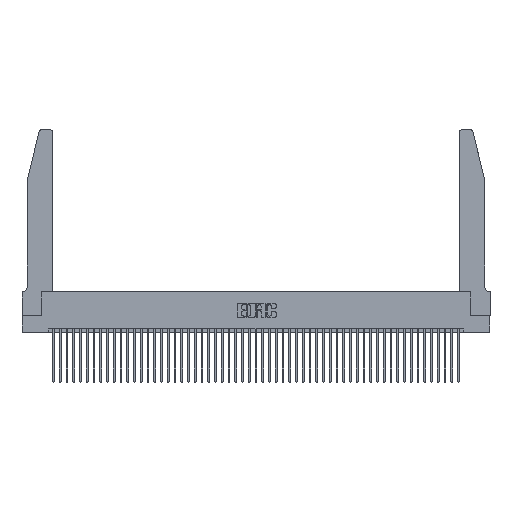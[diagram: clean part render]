
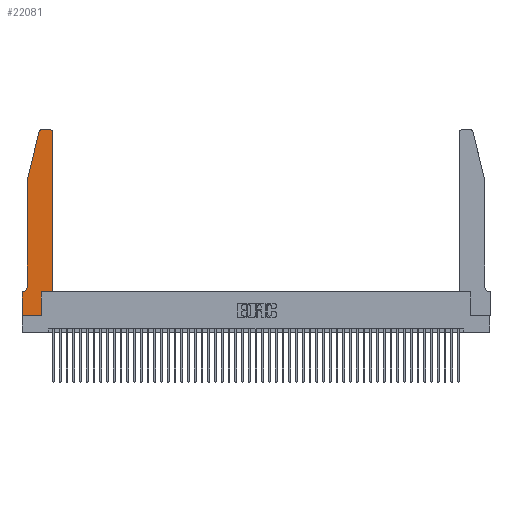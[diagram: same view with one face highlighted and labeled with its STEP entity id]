
A CAD part, top view. The second image highlights one B-rep face of the part: STEP entity #22081.
In plain terms, the highlighted planar face has unit normal (0, 0, 1).
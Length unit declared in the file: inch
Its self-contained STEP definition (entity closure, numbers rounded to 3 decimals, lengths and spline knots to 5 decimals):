
#239 = DIRECTION ( 'NONE',  ( -1., 0., 0. ) ) ;
#537 = CARTESIAN_POINT ( 'NONE',  ( 0.0755, 2., 0.37 ) ) ;
#683 = EDGE_CURVE ( 'NONE', #21842, #46293, #47460, .T. ) ;
#804 = AXIS2_PLACEMENT_3D ( 'NONE', #44240, #5636, #13588 ) ;
#1028 = VERTEX_POINT ( 'NONE', #24618 ) ;
#1749 = VECTOR ( 'NONE', #37568, 39.37008 ) ;
#1905 = EDGE_CURVE ( 'NONE', #1028, #19349, #47567, .T. ) ;
#2103 = ORIENTED_EDGE ( 'NONE', *, *, #21522, .T. ) ;
#2337 = DIRECTION ( 'NONE',  ( 0., 0., 1. ) ) ;
#2637 = CIRCLE ( 'NONE', #40238, 0.03 ) ;
#3831 = VERTEX_POINT ( 'NONE', #17701 ) ;
#4755 = LINE ( 'NONE', #44867, #1749 ) ;
#5112 = CIRCLE ( 'NONE', #804, 0.07 ) ;
#5511 = VECTOR ( 'NONE', #21574, 39.37008 ) ;
#5636 = DIRECTION ( 'NONE',  ( 0., 0., -1. ) ) ;
#5641 = LINE ( 'NONE', #6228, #22602 ) ;
#5674 = VECTOR ( 'NONE', #14822, 39.37008 ) ;
#5679 = CARTESIAN_POINT ( 'NONE',  ( 0.2865, 0.35, 0.37 ) ) ;
#6228 = CARTESIAN_POINT ( 'NONE',  ( 0.4505, 0.35, 0.37 ) ) ;
#7110 = ORIENTED_EDGE ( 'NONE', *, *, #42096, .T. ) ;
#7933 = VERTEX_POINT ( 'NONE', #45067 ) ;
#8116 = VERTEX_POINT ( 'NONE', #537 ) ;
#8693 = ORIENTED_EDGE ( 'NONE', *, *, #1905, .T. ) ;
#8841 = ORIENTED_EDGE ( 'NONE', *, *, #12500, .T. ) ;
#9583 = CARTESIAN_POINT ( 'NONE',  ( 0.4505, 0.35, 0.37 ) ) ;
#9733 = CARTESIAN_POINT ( 'NONE',  ( 0.2865, 0., 0.37 ) ) ;
#9980 = LINE ( 'NONE', #12055, #46241 ) ;
#10110 = VERTEX_POINT ( 'NONE', #5679 ) ;
#10448 = DIRECTION ( 'NONE',  ( 1., 0., 0. ) ) ;
#10725 = CARTESIAN_POINT ( 'NONE',  ( 0., 0.35, 0.37 ) ) ;
#11738 = VECTOR ( 'NONE', #10448, 39.37008 ) ;
#12055 = CARTESIAN_POINT ( 'NONE',  ( 0.0755, 0.35, 0.37 ) ) ;
#12152 = ORIENTED_EDGE ( 'NONE', *, *, #33700, .T. ) ;
#12319 = EDGE_CURVE ( 'NONE', #37560, #8116, #18363, .T. ) ;
#12500 = EDGE_CURVE ( 'NONE', #10110, #3831, #5641, .T. ) ;
#13588 = DIRECTION ( 'NONE',  ( -1., 0., 0. ) ) ;
#13755 = AXIS2_PLACEMENT_3D ( 'NONE', #10725, #14436, #45393 ) ;
#14143 = VECTOR ( 'NONE', #43147, 39.37008 ) ;
#14239 = ORIENTED_EDGE ( 'NONE', *, *, #46675, .T. ) ;
#14299 = LINE ( 'NONE', #9583, #16076 ) ;
#14436 = DIRECTION ( 'NONE',  ( 0., 0., 1. ) ) ;
#14731 = DIRECTION ( 'NONE',  ( 1., 0., 0. ) ) ;
#14822 = DIRECTION ( 'NONE',  ( 0., -1., 0. ) ) ;
#15952 = VERTEX_POINT ( 'NONE', #25430 ) ;
#16050 = CARTESIAN_POINT ( 'NONE',  ( 0.0755, 2., 0.37 ) ) ;
#16076 = VECTOR ( 'NONE', #17682, 39.37008 ) ;
#16560 = CARTESIAN_POINT ( 'NONE',  ( 0.2865, 0.35, 0.37 ) ) ;
#17682 = DIRECTION ( 'NONE',  ( 0., 1., 0. ) ) ;
#17701 = CARTESIAN_POINT ( 'NONE',  ( 0.4505, 0.35, 0.37 ) ) ;
#18363 = LINE ( 'NONE', #16050, #14143 ) ;
#18545 = ORIENTED_EDGE ( 'NONE', *, *, #34803, .T. ) ;
#19349 = VERTEX_POINT ( 'NONE', #48610 ) ;
#21055 = CARTESIAN_POINT ( 'NONE',  ( 0.2605, 2.75, 0.37 ) ) ;
#21522 = EDGE_CURVE ( 'NONE', #8116, #42821, #34781, .T. ) ;
#21574 = DIRECTION ( 'NONE',  ( -1., 0., 0. ) ) ;
#21842 = VERTEX_POINT ( 'NONE', #28499 ) ;
#22081 = ADVANCED_FACE ( 'NONE', ( #41351 ), #49780, .T. ) ;
#22169 = DIRECTION ( 'NONE',  ( 1., 0., 0. ) ) ;
#22558 = CARTESIAN_POINT ( 'NONE',  ( 0.284, 2.75, 0.37 ) ) ;
#22602 = VECTOR ( 'NONE', #37219, 39.37008 ) ;
#24618 = CARTESIAN_POINT ( 'NONE',  ( 0.4505, 2.72, 0.37 ) ) ;
#25430 = CARTESIAN_POINT ( 'NONE',  ( 0., 0.35, 0.37 ) ) ;
#25477 = ORIENTED_EDGE ( 'NONE', *, *, #683, .T. ) ;
#25552 = AXIS2_PLACEMENT_3D ( 'NONE', #41092, #2337, #22169 ) ;
#25712 = DIRECTION ( 'NONE',  ( 0., 1., 0. ) ) ;
#26175 = VERTEX_POINT ( 'NONE', #22558 ) ;
#26187 = CARTESIAN_POINT ( 'NONE',  ( 0., 0., 0.37 ) ) ;
#28037 = EDGE_CURVE ( 'NONE', #19349, #26175, #42472, .T. ) ;
#28499 = CARTESIAN_POINT ( 'NONE',  ( 0., 0., 0.37 ) ) ;
#29831 = LINE ( 'NONE', #16560, #31041 ) ;
#31041 = VECTOR ( 'NONE', #25712, 39.37008 ) ;
#31702 = EDGE_LOOP ( 'NONE', ( #41943, #38095, #37378, #2103, #18545, #14239, #35627, #25477, #12152, #8841, #7110, #8693 ) ) ;
#33700 = EDGE_CURVE ( 'NONE', #46293, #10110, #29831, .T. ) ;
#34781 = LINE ( 'NONE', #37824, #5674 ) ;
#34803 = EDGE_CURVE ( 'NONE', #42821, #7933, #5112, .T. ) ;
#35627 = ORIENTED_EDGE ( 'NONE', *, *, #48281, .T. ) ;
#37219 = DIRECTION ( 'NONE',  ( 1., 0., 0. ) ) ;
#37378 = ORIENTED_EDGE ( 'NONE', *, *, #12319, .T. ) ;
#37560 = VERTEX_POINT ( 'NONE', #38539 ) ;
#37568 = DIRECTION ( 'NONE',  ( 0., -1., 0. ) ) ;
#37824 = CARTESIAN_POINT ( 'NONE',  ( 0.0755, 2., 0.37 ) ) ;
#38095 = ORIENTED_EDGE ( 'NONE', *, *, #43535, .T. ) ;
#38539 = CARTESIAN_POINT ( 'NONE',  ( 0.25487, 2.72718, 0.37 ) ) ;
#38951 = CARTESIAN_POINT ( 'NONE',  ( 0.0755, 0.42, 0.37 ) ) ;
#40238 = AXIS2_PLACEMENT_3D ( 'NONE', #45844, #50053, #14731 ) ;
#41092 = CARTESIAN_POINT ( 'NONE',  ( 0.4205, 2.72, 0.37 ) ) ;
#41351 = FACE_OUTER_BOUND ( 'NONE', #31702, .T. ) ;
#41943 = ORIENTED_EDGE ( 'NONE', *, *, #28037, .T. ) ;
#42096 = EDGE_CURVE ( 'NONE', #3831, #1028, #14299, .T. ) ;
#42472 = LINE ( 'NONE', #21055, #5511 ) ;
#42821 = VERTEX_POINT ( 'NONE', #38951 ) ;
#43147 = DIRECTION ( 'NONE',  ( -0.239, -0.971, 0. ) ) ;
#43535 = EDGE_CURVE ( 'NONE', #26175, #37560, #2637, .T. ) ;
#44240 = CARTESIAN_POINT ( 'NONE',  ( 0.0055, 0.42, 0.37 ) ) ;
#44867 = CARTESIAN_POINT ( 'NONE',  ( 0., 0., 0.37 ) ) ;
#45067 = CARTESIAN_POINT ( 'NONE',  ( 0.0055, 0.35, 0.37 ) ) ;
#45393 = DIRECTION ( 'NONE',  ( 1., 0., 0. ) ) ;
#45844 = CARTESIAN_POINT ( 'NONE',  ( 0.284, 2.72, 0.37 ) ) ;
#46241 = VECTOR ( 'NONE', #239, 39.37008 ) ;
#46293 = VERTEX_POINT ( 'NONE', #9733 ) ;
#46675 = EDGE_CURVE ( 'NONE', #7933, #15952, #9980, .T. ) ;
#47460 = LINE ( 'NONE', #26187, #11738 ) ;
#47567 = CIRCLE ( 'NONE', #25552, 0.03 ) ;
#48281 = EDGE_CURVE ( 'NONE', #15952, #21842, #4755, .T. ) ;
#48610 = CARTESIAN_POINT ( 'NONE',  ( 0.4205, 2.75, 0.37 ) ) ;
#49780 = PLANE ( 'NONE',  #13755 ) ;
#50053 = DIRECTION ( 'NONE',  ( 0., 0., 1. ) ) ;
